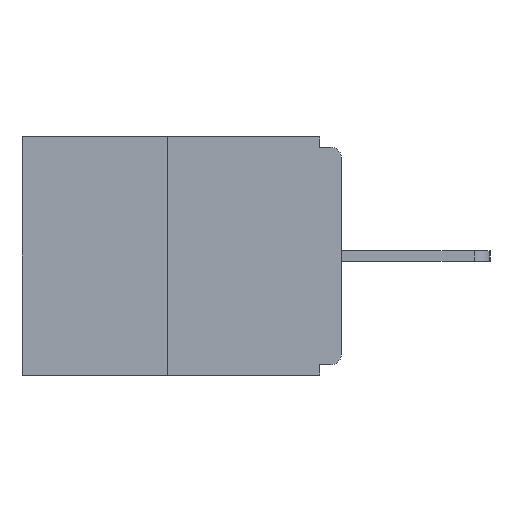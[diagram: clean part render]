
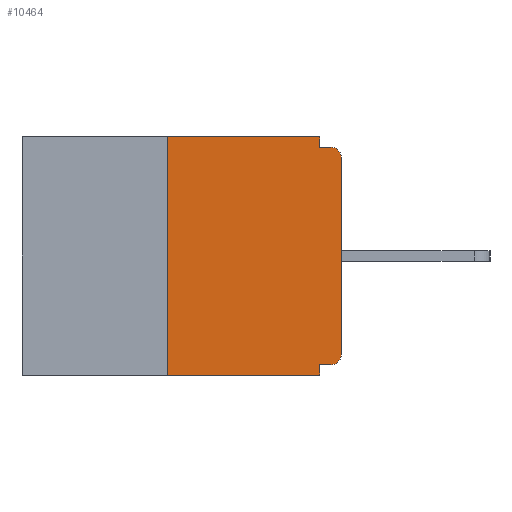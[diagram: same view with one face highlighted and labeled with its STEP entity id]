
A CAD part, left-side view. The second image highlights one B-rep face of the part: STEP entity #10464.
In plain terms, the highlighted planar face has unit normal (-1, 0, 0).
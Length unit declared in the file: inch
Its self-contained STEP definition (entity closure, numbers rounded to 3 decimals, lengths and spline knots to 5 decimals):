
#69 = EDGE_CURVE ( 'NONE', #2128, #8253, #1002, .T. ) ;
#88 = DIRECTION ( 'NONE',  ( 0., -1., 0. ) ) ;
#108 = EDGE_CURVE ( 'NONE', #7351, #3312, #8755, .T. ) ;
#239 = VECTOR ( 'NONE', #10944, 39.37008 ) ;
#263 = VERTEX_POINT ( 'NONE', #9821 ) ;
#594 = CARTESIAN_POINT ( 'NONE',  ( 0., 0.015, -0.015 ) ) ;
#762 = DIRECTION ( 'NONE',  ( 0., 0., 1. ) ) ;
#1002 = LINE ( 'NONE', #2112, #2962 ) ;
#1011 = AXIS2_PLACEMENT_3D ( 'NONE', #5845, #2146, #3142 ) ;
#1034 = DIRECTION ( 'NONE',  ( 0., 1., 0. ) ) ;
#1076 = LINE ( 'NONE', #8566, #7780 ) ;
#1515 = CARTESIAN_POINT ( 'NONE',  ( 0., 0.031, -0.343 ) ) ;
#1705 = EDGE_CURVE ( 'NONE', #2204, #3312, #11513, .T. ) ;
#1899 = ORIENTED_EDGE ( 'NONE', *, *, #11371, .T. ) ;
#2017 = LINE ( 'NONE', #3749, #4262 ) ;
#2026 = EDGE_CURVE ( 'NONE', #3269, #2204, #2017, .T. ) ;
#2112 = CARTESIAN_POINT ( 'NONE',  ( 0., 0., -0.015 ) ) ;
#2128 = VERTEX_POINT ( 'NONE', #7903 ) ;
#2146 = DIRECTION ( 'NONE',  ( -1., 0., 0. ) ) ;
#2160 = DIRECTION ( 'NONE',  ( 0., 0., -1. ) ) ;
#2204 = VERTEX_POINT ( 'NONE', #5158 ) ;
#2282 = PLANE ( 'NONE',  #4610 ) ;
#2380 = CIRCLE ( 'NONE', #3937, 0.015 ) ;
#2699 = EDGE_CURVE ( 'NONE', #7351, #8386, #10244, .T. ) ;
#2962 = VECTOR ( 'NONE', #9627, 39.37008 ) ;
#3035 = CARTESIAN_POINT ( 'NONE',  ( 0., 0.031, -0.343 ) ) ;
#3142 = DIRECTION ( 'NONE',  ( 0., 0., -1. ) ) ;
#3184 = ORIENTED_EDGE ( 'NONE', *, *, #69, .F. ) ;
#3203 = ORIENTED_EDGE ( 'NONE', *, *, #2699, .F. ) ;
#3269 = VERTEX_POINT ( 'NONE', #11695 ) ;
#3312 = VERTEX_POINT ( 'NONE', #1515 ) ;
#3524 = DIRECTION ( 'NONE',  ( 0., 0., -1. ) ) ;
#3593 = CARTESIAN_POINT ( 'NONE',  ( 0., 0.25, -0.343 ) ) ;
#3742 = ORIENTED_EDGE ( 'NONE', *, *, #5693, .T. ) ;
#3749 = CARTESIAN_POINT ( 'NONE',  ( 0., 0., -0.328 ) ) ;
#3845 = CARTESIAN_POINT ( 'NONE',  ( 0., 0.25, 0. ) ) ;
#3857 = VECTOR ( 'NONE', #2160, 39.37008 ) ;
#3937 = AXIS2_PLACEMENT_3D ( 'NONE', #10107, #5363, #3524 ) ;
#4068 = DIRECTION ( 'NONE',  ( 0., 0., -1. ) ) ;
#4125 = LINE ( 'NONE', #5859, #9184 ) ;
#4262 = VECTOR ( 'NONE', #1034, 39.37008 ) ;
#4356 = CIRCLE ( 'NONE', #1011, 0.015 ) ;
#4541 = CARTESIAN_POINT ( 'NONE',  ( 0., 0., -0.03 ) ) ;
#4610 = AXIS2_PLACEMENT_3D ( 'NONE', #11567, #10591, #7786 ) ;
#4818 = ORIENTED_EDGE ( 'NONE', *, *, #9269, .T. ) ;
#5038 = VECTOR ( 'NONE', #762, 39.37008 ) ;
#5158 = CARTESIAN_POINT ( 'NONE',  ( 0., 0.031, -0.328 ) ) ;
#5363 = DIRECTION ( 'NONE',  ( -1., 0., 0. ) ) ;
#5693 = EDGE_CURVE ( 'NONE', #6509, #8253, #2380, .T. ) ;
#5845 = CARTESIAN_POINT ( 'NONE',  ( 0., 0.015, -0.313 ) ) ;
#5859 = CARTESIAN_POINT ( 'NONE',  ( 0., 0.031, 0. ) ) ;
#6089 = FACE_OUTER_BOUND ( 'NONE', #8327, .T. ) ;
#6099 = ORIENTED_EDGE ( 'NONE', *, *, #7206, .F. ) ;
#6509 = VERTEX_POINT ( 'NONE', #4541 ) ;
#6689 = CARTESIAN_POINT ( 'NONE',  ( 0., 0.46, -0.343 ) ) ;
#7206 = EDGE_CURVE ( 'NONE', #8386, #9682, #1076, .T. ) ;
#7351 = VERTEX_POINT ( 'NONE', #3593 ) ;
#7646 = EDGE_CURVE ( 'NONE', #9682, #2128, #4125, .T. ) ;
#7780 = VECTOR ( 'NONE', #88, 39.37008 ) ;
#7786 = DIRECTION ( 'NONE',  ( 0., 0., -1. ) ) ;
#7903 = CARTESIAN_POINT ( 'NONE',  ( 0., 0.031, -0.015 ) ) ;
#8242 = ORIENTED_EDGE ( 'NONE', *, *, #108, .T. ) ;
#8253 = VERTEX_POINT ( 'NONE', #594 ) ;
#8327 = EDGE_LOOP ( 'NONE', ( #6099, #3203, #8242, #8653, #9294, #4818, #1899, #3742, #3184, #11280 ) ) ;
#8386 = VERTEX_POINT ( 'NONE', #3845 ) ;
#8559 = DIRECTION ( 'NONE',  ( 0., -1., 0. ) ) ;
#8566 = CARTESIAN_POINT ( 'NONE',  ( 0., 0.46, 0. ) ) ;
#8653 = ORIENTED_EDGE ( 'NONE', *, *, #1705, .F. ) ;
#8755 = LINE ( 'NONE', #6689, #8904 ) ;
#8904 = VECTOR ( 'NONE', #8559, 39.37008 ) ;
#9184 = VECTOR ( 'NONE', #4068, 39.37008 ) ;
#9269 = EDGE_CURVE ( 'NONE', #3269, #263, #4356, .T. ) ;
#9294 = ORIENTED_EDGE ( 'NONE', *, *, #2026, .F. ) ;
#9383 = LINE ( 'NONE', #10025, #239 ) ;
#9627 = DIRECTION ( 'NONE',  ( 0., -1., 0. ) ) ;
#9682 = VERTEX_POINT ( 'NONE', #10122 ) ;
#9821 = CARTESIAN_POINT ( 'NONE',  ( 0., 0., -0.313 ) ) ;
#10025 = CARTESIAN_POINT ( 'NONE',  ( 0., 0., 0. ) ) ;
#10107 = CARTESIAN_POINT ( 'NONE',  ( 0., 0.015, -0.03 ) ) ;
#10122 = CARTESIAN_POINT ( 'NONE',  ( 0., 0.031, 0. ) ) ;
#10244 = LINE ( 'NONE', #11156, #5038 ) ;
#10464 = ADVANCED_FACE ( 'NONE', ( #6089 ), #2282, .F. ) ;
#10591 = DIRECTION ( 'NONE',  ( 1., 0., 0. ) ) ;
#10944 = DIRECTION ( 'NONE',  ( 0., 0., 1. ) ) ;
#11156 = CARTESIAN_POINT ( 'NONE',  ( 0., 0.25, 0. ) ) ;
#11280 = ORIENTED_EDGE ( 'NONE', *, *, #7646, .F. ) ;
#11371 = EDGE_CURVE ( 'NONE', #263, #6509, #9383, .T. ) ;
#11513 = LINE ( 'NONE', #3035, #3857 ) ;
#11567 = CARTESIAN_POINT ( 'NONE',  ( 0., 0.46, 0. ) ) ;
#11695 = CARTESIAN_POINT ( 'NONE',  ( 0., 0.015, -0.328 ) ) ;
